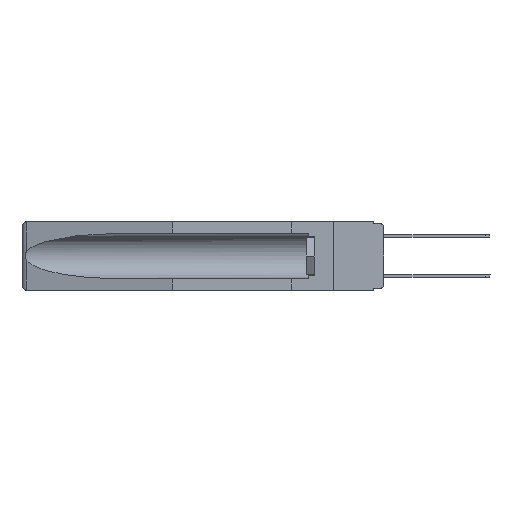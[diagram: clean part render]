
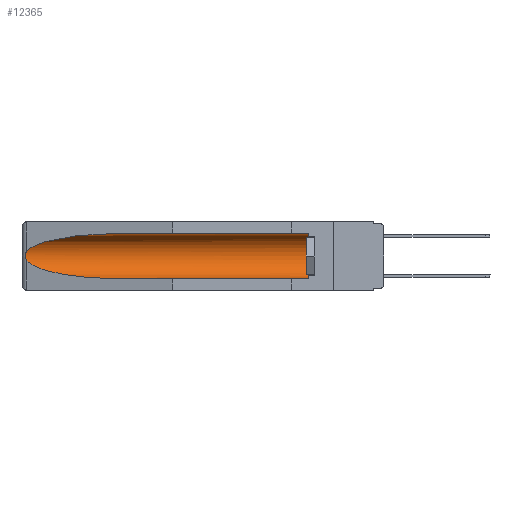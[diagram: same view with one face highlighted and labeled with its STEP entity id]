
A CAD part, left-side view. The second image highlights one B-rep face of the part: STEP entity #12365.
In plain terms, the highlighted cylindrical face has radius 2.857 mm (diameter 5.715 mm), a partial arc.
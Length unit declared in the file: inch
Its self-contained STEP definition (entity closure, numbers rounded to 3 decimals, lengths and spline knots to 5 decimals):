
#201 = ORIENTED_EDGE ( 'NONE', *, *, #13275, .T. ) ;
#400 = EDGE_CURVE ( 'NONE', #1056, #17009, #17631, .T. ) ;
#511 = CARTESIAN_POINT ( 'NONE',  ( 0.26597, 1.5296, -0.19026 ) ) ;
#602 = CARTESIAN_POINT ( 'NONE',  ( 0.2675, 1.53308, -0.16763 ) ) ;
#1056 = VERTEX_POINT ( 'NONE', #18085 ) ;
#1253 = CARTESIAN_POINT ( 'NONE',  ( 0.155, 1.07973, -0.284 ) ) ;
#1400 = CARTESIAN_POINT ( 'NONE',  ( 0.26537, 1.52718, -0.14972 ) ) ;
#1467 = CARTESIAN_POINT ( 'NONE',  ( 0.155, 0.126, -0.284 ) ) ;
#1512 = CARTESIAN_POINT ( 'NONE',  ( 0.26537, 1.52718, -0.19328 ) ) ;
#1566 = EDGE_CURVE ( 'NONE', #12660, #12231, #9685, .T. ) ;
#1828 = ORIENTED_EDGE ( 'NONE', *, *, #7103, .F. ) ;
#1846 = CARTESIAN_POINT ( 'NONE',  ( 0.155, -0.30754, -0.1715 ) ) ;
#1980 = CARTESIAN_POINT ( 'NONE',  ( 0.26597, 1.52961, -0.15275 ) ) ;
#2208 = DIRECTION ( 'NONE',  ( 0., 0., 1. ) ) ;
#2629 = CARTESIAN_POINT ( 'NONE',  ( 0.26537, 1.52718, -0.19328 ) ) ;
#2878 = EDGE_CURVE ( 'NONE', #12231, #15595, #8649, .T. ) ;
#3097 = DIRECTION ( 'NONE',  ( 0., -1., 0. ) ) ;
#3328 = DIRECTION ( 'NONE',  ( 0., 1., 0. ) ) ;
#4029 = AXIS2_PLACEMENT_3D ( 'NONE', #17307, #3097, #10255 ) ;
#4160 = CARTESIAN_POINT ( 'NONE',  ( 0.155, 1.07973, -0.059 ) ) ;
#4323 =( BOUNDED_CURVE ( )  B_SPLINE_CURVE ( 3, ( #4160, #8440, #18291, #1400 ),
 .UNSPECIFIED., .F., .F. ) 
 B_SPLINE_CURVE_WITH_KNOTS ( ( 4, 4 ),
 ( 4.71239, 6.08839 ),
 .UNSPECIFIED. ) 
 CURVE ( )  GEOMETRIC_REPRESENTATION_ITEM ( )  RATIONAL_B_SPLINE_CURVE ( ( 1., 0.848, 0.848, 1. ) ) 
 REPRESENTATION_ITEM ( '' )  );
#4654 = VECTOR ( 'NONE', #14319, 39.37008 ) ;
#4831 = CARTESIAN_POINT ( 'NONE',  ( 0.26654, 1.53092, -0.15636 ) ) ;
#5504 = VECTOR ( 'NONE', #3328, 39.37008 ) ;
#6091 = DIRECTION ( 'NONE',  ( 0., 1., 0. ) ) ;
#6111 = CARTESIAN_POINT ( 'NONE',  ( 0.155, -0.30754, -0.284 ) ) ;
#6960 = ORIENTED_EDGE ( 'NONE', *, *, #400, .T. ) ;
#7103 = EDGE_CURVE ( 'NONE', #12660, #14367, #7510, .T. ) ;
#7510 = LINE ( 'NONE', #6111, #5504 ) ;
#7536 =( BOUNDED_CURVE ( )  B_SPLINE_CURVE ( 3, ( #2629, #14137, #17012, #1253 ),
 .UNSPECIFIED., .F., .F. ) 
 B_SPLINE_CURVE_WITH_KNOTS ( ( 4, 4 ),
 ( 0.1948, 1.5708 ),
 .UNSPECIFIED. ) 
 CURVE ( )  GEOMETRIC_REPRESENTATION_ITEM ( )  RATIONAL_B_SPLINE_CURVE ( ( 1., 0.848, 0.848, 1. ) ) 
 REPRESENTATION_ITEM ( '' )  );
#7635 = CARTESIAN_POINT ( 'NONE',  ( 0.26537, 1.52718, -0.19328 ) ) ;
#7819 = CARTESIAN_POINT ( 'NONE',  ( 0.2673, 1.53269, -0.17917 ) ) ;
#8440 = CARTESIAN_POINT ( 'NONE',  ( 0.21114, 1.30732, -0.059 ) ) ;
#8649 = LINE ( 'NONE', #10237, #4654 ) ;
#9685 = CIRCLE ( 'NONE', #4029, 0.1125 ) ;
#10188 = ORIENTED_EDGE ( 'NONE', *, *, #1566, .T. ) ;
#10237 = CARTESIAN_POINT ( 'NONE',  ( 0.155, -0.30754, -0.059 ) ) ;
#10255 = DIRECTION ( 'NONE',  ( 0., 0., 1. ) ) ;
#10876 = ORIENTED_EDGE ( 'NONE', *, *, #12923, .T. ) ;
#10920 = CARTESIAN_POINT ( 'NONE',  ( 0.155, 1.07973, -0.284 ) ) ;
#12054 = FACE_OUTER_BOUND ( 'NONE', #13582, .T. ) ;
#12114 = CARTESIAN_POINT ( 'NONE',  ( 0.2673, 1.5327, -0.16383 ) ) ;
#12231 = VERTEX_POINT ( 'NONE', #12913 ) ;
#12365 = ADVANCED_FACE ( 'NONE', ( #12054 ), #17810, .F. ) ;
#12660 = VERTEX_POINT ( 'NONE', #1467 ) ;
#12913 = CARTESIAN_POINT ( 'NONE',  ( 0.155, 0.126, -0.059 ) ) ;
#12923 = EDGE_CURVE ( 'NONE', #17009, #14367, #7536, .T. ) ;
#13254 = AXIS2_PLACEMENT_3D ( 'NONE', #1846, #6091, #2208 ) ;
#13275 = EDGE_CURVE ( 'NONE', #15595, #1056, #4323, .T. ) ;
#13334 = CARTESIAN_POINT ( 'NONE',  ( 0.26537, 1.52718, -0.14972 ) ) ;
#13582 = EDGE_LOOP ( 'NONE', ( #201, #6960, #10876, #1828, #10188, #16600 ) ) ;
#14137 = CARTESIAN_POINT ( 'NONE',  ( 0.25451, 1.48313, -0.24835 ) ) ;
#14319 = DIRECTION ( 'NONE',  ( 0., 1., 0. ) ) ;
#14367 = VERTEX_POINT ( 'NONE', #10920 ) ;
#14790 = CARTESIAN_POINT ( 'NONE',  ( 0.2675, 1.53308, -0.17534 ) ) ;
#15054 = CARTESIAN_POINT ( 'NONE',  ( 0.155, 1.07973, -0.059 ) ) ;
#15595 = VERTEX_POINT ( 'NONE', #15054 ) ;
#16600 = ORIENTED_EDGE ( 'NONE', *, *, #2878, .T. ) ;
#17009 = VERTEX_POINT ( 'NONE', #1512 ) ;
#17012 = CARTESIAN_POINT ( 'NONE',  ( 0.21114, 1.30732, -0.284 ) ) ;
#17307 = CARTESIAN_POINT ( 'NONE',  ( 0.155, 0.126, -0.1715 ) ) ;
#17631 = B_SPLINE_CURVE_WITH_KNOTS ( 'NONE', 3,
 ( #13334, #1980, #4831, #12114, #602, #14790, #7819, #17671, #511, #7635 ),
 .UNSPECIFIED., .F., .F.,
 ( 4, 2, 2, 2, 4 ),
 ( 0., 0.00029, 0.00058, 0.00087, 0.00117 ),
 .UNSPECIFIED. ) ;
#17671 = CARTESIAN_POINT ( 'NONE',  ( 0.26655, 1.53094, -0.18657 ) ) ;
#17810 = CYLINDRICAL_SURFACE ( 'NONE', #13254, 0.1125 ) ;
#18085 = CARTESIAN_POINT ( 'NONE',  ( 0.26537, 1.52718, -0.14972 ) ) ;
#18291 = CARTESIAN_POINT ( 'NONE',  ( 0.25451, 1.48313, -0.09465 ) ) ;
